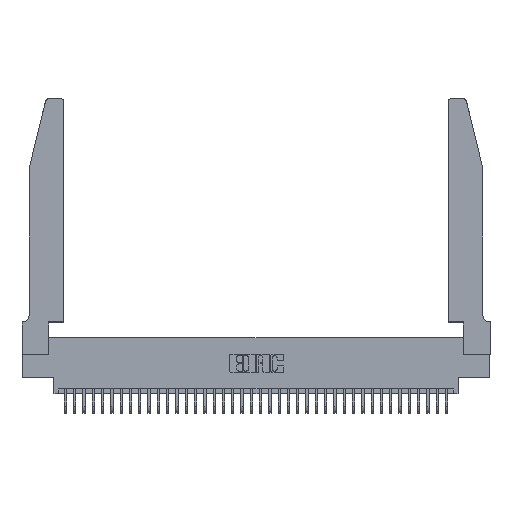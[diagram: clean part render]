
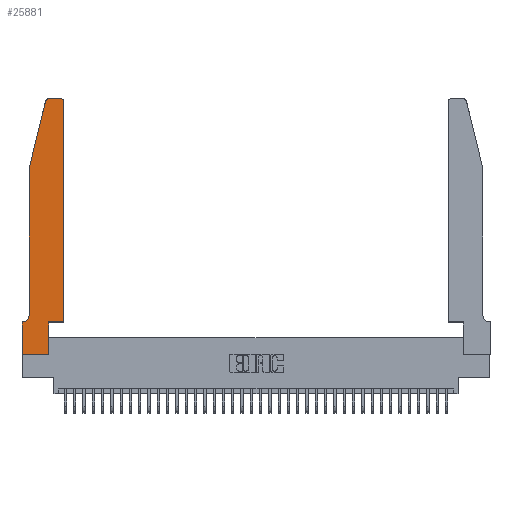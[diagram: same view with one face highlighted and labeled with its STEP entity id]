
A CAD part, top view. The second image highlights one B-rep face of the part: STEP entity #25881.
In plain terms, the highlighted planar face has unit normal (0, 0, 1).
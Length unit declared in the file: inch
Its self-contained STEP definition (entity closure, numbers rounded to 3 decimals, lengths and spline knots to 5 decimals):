
#559 = VERTEX_POINT ( 'NONE', #15111 ) ;
#795 = CARTESIAN_POINT ( 'NONE',  ( 0.4505, 0.35, 0.37 ) ) ;
#1120 = ORIENTED_EDGE ( 'NONE', *, *, #38236, .T. ) ;
#1711 = CARTESIAN_POINT ( 'NONE',  ( 0.4505, 0.35, 0.37 ) ) ;
#1835 = VECTOR ( 'NONE', #3326, 39.37008 ) ;
#2495 = VERTEX_POINT ( 'NONE', #15474 ) ;
#3018 = DIRECTION ( 'NONE',  ( 1., 0., 0. ) ) ;
#3178 = DIRECTION ( 'NONE',  ( 0., 0., 1. ) ) ;
#3260 = ORIENTED_EDGE ( 'NONE', *, *, #32755, .T. ) ;
#3326 = DIRECTION ( 'NONE',  ( 0., -1., 0. ) ) ;
#3642 = ORIENTED_EDGE ( 'NONE', *, *, #25996, .T. ) ;
#3958 = AXIS2_PLACEMENT_3D ( 'NONE', #15562, #33556, #33441 ) ;
#4984 = CARTESIAN_POINT ( 'NONE',  ( 0.4505, 0.35, 0.37 ) ) ;
#5029 = ORIENTED_EDGE ( 'NONE', *, *, #18987, .T. ) ;
#5072 = DIRECTION ( 'NONE',  ( 1., 0., 0. ) ) ;
#5262 = DIRECTION ( 'NONE',  ( 0., 1., 0. ) ) ;
#5469 = EDGE_CURVE ( 'NONE', #22794, #11568, #15050, .T. ) ;
#5943 = AXIS2_PLACEMENT_3D ( 'NONE', #30775, #3178, #33831 ) ;
#6447 = VERTEX_POINT ( 'NONE', #20490 ) ;
#6487 = CARTESIAN_POINT ( 'NONE',  ( 0., 0.35, 0.37 ) ) ;
#6634 = CARTESIAN_POINT ( 'NONE',  ( 0., 0., 0.37 ) ) ;
#6971 = CARTESIAN_POINT ( 'NONE',  ( 0.0755, 0.35, 0.37 ) ) ;
#7460 = LINE ( 'NONE', #7467, #13667 ) ;
#7467 = CARTESIAN_POINT ( 'NONE',  ( 0., 0., 0.37 ) ) ;
#7928 = LINE ( 'NONE', #4984, #8924 ) ;
#8132 = VERTEX_POINT ( 'NONE', #12016 ) ;
#8316 = CARTESIAN_POINT ( 'NONE',  ( 0.2605, 2.75, 0.37 ) ) ;
#8528 = VERTEX_POINT ( 'NONE', #15958 ) ;
#8924 = VECTOR ( 'NONE', #5262, 39.37008 ) ;
#9819 = ORIENTED_EDGE ( 'NONE', *, *, #18039, .T. ) ;
#10003 = DIRECTION ( 'NONE',  ( -1., 0., 0. ) ) ;
#10916 = CARTESIAN_POINT ( 'NONE',  ( 0.284, 2.75, 0.37 ) ) ;
#11033 = CARTESIAN_POINT ( 'NONE',  ( 0.0055, 0.35, 0.37 ) ) ;
#11418 = CARTESIAN_POINT ( 'NONE',  ( 0.25487, 2.72718, 0.37 ) ) ;
#11568 = VERTEX_POINT ( 'NONE', #10916 ) ;
#11862 = PLANE ( 'NONE',  #32061 ) ;
#12016 = CARTESIAN_POINT ( 'NONE',  ( 0.0755, 0.42, 0.37 ) ) ;
#12927 = VERTEX_POINT ( 'NONE', #11033 ) ;
#13265 = CARTESIAN_POINT ( 'NONE',  ( 0., 0., 0.37 ) ) ;
#13667 = VECTOR ( 'NONE', #25507, 39.37008 ) ;
#13751 = DIRECTION ( 'NONE',  ( -1., 0., 0. ) ) ;
#14109 = CARTESIAN_POINT ( 'NONE',  ( 0.4205, 2.75, 0.37 ) ) ;
#14335 = CIRCLE ( 'NONE', #26507, 0.03 ) ;
#15050 = LINE ( 'NONE', #8316, #34097 ) ;
#15111 = CARTESIAN_POINT ( 'NONE',  ( 0.2865, 0.35, 0.37 ) ) ;
#15337 = LINE ( 'NONE', #37263, #20123 ) ;
#15380 = LINE ( 'NONE', #13265, #23010 ) ;
#15474 = CARTESIAN_POINT ( 'NONE',  ( 0.0755, 2., 0.37 ) ) ;
#15562 = CARTESIAN_POINT ( 'NONE',  ( 0.0055, 0.42, 0.37 ) ) ;
#15958 = CARTESIAN_POINT ( 'NONE',  ( 0.4505, 2.72, 0.37 ) ) ;
#17267 = CARTESIAN_POINT ( 'NONE',  ( 0.4205, 2.72, 0.37 ) ) ;
#17926 = EDGE_CURVE ( 'NONE', #2495, #8132, #26731, .T. ) ;
#18039 = EDGE_CURVE ( 'NONE', #12927, #26004, #22875, .T. ) ;
#18095 = ORIENTED_EDGE ( 'NONE', *, *, #29818, .T. ) ;
#18532 = CIRCLE ( 'NONE', #5943, 0.03 ) ;
#18973 = FACE_OUTER_BOUND ( 'NONE', #36728, .T. ) ;
#18987 = EDGE_CURVE ( 'NONE', #19254, #6447, #7460, .T. ) ;
#19220 = ORIENTED_EDGE ( 'NONE', *, *, #22866, .T. ) ;
#19254 = VERTEX_POINT ( 'NONE', #6634 ) ;
#20123 = VECTOR ( 'NONE', #34323, 39.37008 ) ;
#20490 = CARTESIAN_POINT ( 'NONE',  ( 0.2865, 0., 0.37 ) ) ;
#21464 = ORIENTED_EDGE ( 'NONE', *, *, #26443, .T. ) ;
#21733 = CARTESIAN_POINT ( 'NONE',  ( 0., 0.35, 0.37 ) ) ;
#21801 = VERTEX_POINT ( 'NONE', #795 ) ;
#22247 = DIRECTION ( 'NONE',  ( 0., -1., 0. ) ) ;
#22794 = VERTEX_POINT ( 'NONE', #14109 ) ;
#22866 = EDGE_CURVE ( 'NONE', #6447, #559, #25824, .T. ) ;
#22875 = LINE ( 'NONE', #6971, #33828 ) ;
#22960 = VECTOR ( 'NONE', #33391, 39.37008 ) ;
#23010 = VECTOR ( 'NONE', #22247, 39.37008 ) ;
#23063 = EDGE_CURVE ( 'NONE', #559, #21801, #37222, .T. ) ;
#23216 = ORIENTED_EDGE ( 'NONE', *, *, #37954, .T. ) ;
#24323 = ORIENTED_EDGE ( 'NONE', *, *, #23063, .T. ) ;
#25366 = VECTOR ( 'NONE', #5072, 39.37008 ) ;
#25507 = DIRECTION ( 'NONE',  ( 1., 0., 0. ) ) ;
#25824 = LINE ( 'NONE', #28186, #22960 ) ;
#25881 = ADVANCED_FACE ( 'NONE', ( #18973 ), #11862, .T. ) ;
#25996 = EDGE_CURVE ( 'NONE', #8132, #12927, #39008, .T. ) ;
#26004 = VERTEX_POINT ( 'NONE', #21733 ) ;
#26443 = EDGE_CURVE ( 'NONE', #21801, #8528, #7928, .T. ) ;
#26507 = AXIS2_PLACEMENT_3D ( 'NONE', #17267, #39128, #38732 ) ;
#26731 = LINE ( 'NONE', #30560, #1835 ) ;
#27217 = ORIENTED_EDGE ( 'NONE', *, *, #17926, .T. ) ;
#27821 = DIRECTION ( 'NONE',  ( 0., 0., 1. ) ) ;
#28186 = CARTESIAN_POINT ( 'NONE',  ( 0.2865, 0.35, 0.37 ) ) ;
#29818 = EDGE_CURVE ( 'NONE', #26004, #19254, #15380, .T. ) ;
#30227 = VERTEX_POINT ( 'NONE', #11418 ) ;
#30560 = CARTESIAN_POINT ( 'NONE',  ( 0.0755, 2., 0.37 ) ) ;
#30775 = CARTESIAN_POINT ( 'NONE',  ( 0.284, 2.72, 0.37 ) ) ;
#32061 = AXIS2_PLACEMENT_3D ( 'NONE', #6487, #27821, #3018 ) ;
#32755 = EDGE_CURVE ( 'NONE', #11568, #30227, #18532, .T. ) ;
#33391 = DIRECTION ( 'NONE',  ( 0., 1., 0. ) ) ;
#33441 = DIRECTION ( 'NONE',  ( -1., 0., 0. ) ) ;
#33556 = DIRECTION ( 'NONE',  ( 0., 0., -1. ) ) ;
#33828 = VECTOR ( 'NONE', #10003, 39.37008 ) ;
#33831 = DIRECTION ( 'NONE',  ( 1., 0., 0. ) ) ;
#34097 = VECTOR ( 'NONE', #13751, 39.37008 ) ;
#34323 = DIRECTION ( 'NONE',  ( -0.239, -0.971, 0. ) ) ;
#36728 = EDGE_LOOP ( 'NONE', ( #36815, #3260, #23216, #27217, #3642, #9819, #18095, #5029, #19220, #24323, #21464, #1120 ) ) ;
#36815 = ORIENTED_EDGE ( 'NONE', *, *, #5469, .T. ) ;
#37222 = LINE ( 'NONE', #1711, #25366 ) ;
#37263 = CARTESIAN_POINT ( 'NONE',  ( 0.0755, 2., 0.37 ) ) ;
#37954 = EDGE_CURVE ( 'NONE', #30227, #2495, #15337, .T. ) ;
#38236 = EDGE_CURVE ( 'NONE', #8528, #22794, #14335, .T. ) ;
#38732 = DIRECTION ( 'NONE',  ( 1., 0., 0. ) ) ;
#39008 = CIRCLE ( 'NONE', #3958, 0.07 ) ;
#39128 = DIRECTION ( 'NONE',  ( 0., 0., 1. ) ) ;
